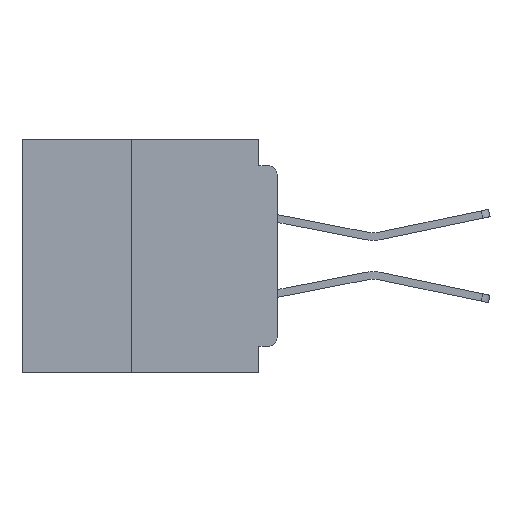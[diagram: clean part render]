
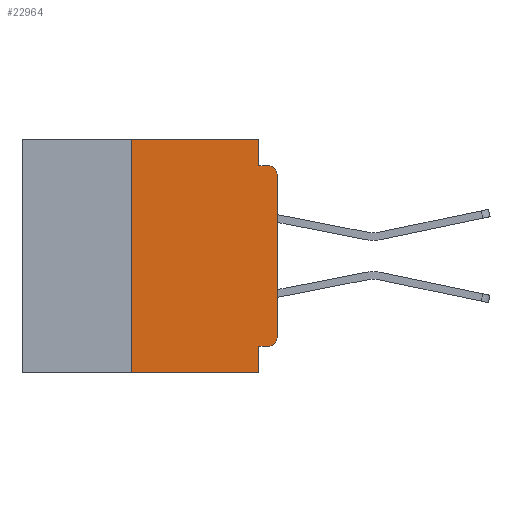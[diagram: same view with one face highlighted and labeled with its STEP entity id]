
A CAD part, left-side view. The second image highlights one B-rep face of the part: STEP entity #22964.
In plain terms, the highlighted planar face has unit normal (-1, 0, 0).
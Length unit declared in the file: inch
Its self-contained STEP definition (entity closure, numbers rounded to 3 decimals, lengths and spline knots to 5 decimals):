
#797 = ORIENTED_EDGE ( 'NONE', *, *, #20829, .T. ) ;
#1443 = DIRECTION ( 'NONE',  ( -1., 0., 0. ) ) ;
#1521 = VERTEX_POINT ( 'NONE', #8907 ) ;
#2246 = CARTESIAN_POINT ( 'NONE',  ( 0., 0.25, 0. ) ) ;
#2612 = FACE_OUTER_BOUND ( 'NONE', #40411, .T. ) ;
#3037 = DIRECTION ( 'NONE',  ( 0., 0., -1. ) ) ;
#3996 = CARTESIAN_POINT ( 'NONE',  ( 0., 0.25, -0.4 ) ) ;
#4849 = CARTESIAN_POINT ( 'NONE',  ( 0., 0.437, 0. ) ) ;
#5281 = VERTEX_POINT ( 'NONE', #40898 ) ;
#5335 = AXIS2_PLACEMENT_3D ( 'NONE', #21804, #1443, #25187 ) ;
#5814 = ORIENTED_EDGE ( 'NONE', *, *, #21959, .T. ) ;
#6691 = LINE ( 'NONE', #37808, #23656 ) ;
#6811 = LINE ( 'NONE', #42361, #14792 ) ;
#7474 = VERTEX_POINT ( 'NONE', #8950 ) ;
#7565 = CARTESIAN_POINT ( 'NONE',  ( 0., 0.031, 0. ) ) ;
#8783 = CARTESIAN_POINT ( 'NONE',  ( 0., 0.015, -0.06 ) ) ;
#8907 = CARTESIAN_POINT ( 'NONE',  ( 0., 0.25, -0.4 ) ) ;
#8950 = CARTESIAN_POINT ( 'NONE',  ( 0., 0.031, 0. ) ) ;
#9202 = VECTOR ( 'NONE', #11001, 39.37008 ) ;
#9254 = CARTESIAN_POINT ( 'NONE',  ( 0., 0.437, -0.4 ) ) ;
#9790 = LINE ( 'NONE', #35557, #41506 ) ;
#11001 = DIRECTION ( 'NONE',  ( 0., 0., -1. ) ) ;
#12199 = DIRECTION ( 'NONE',  ( 0., 0., -1. ) ) ;
#14130 = CARTESIAN_POINT ( 'NONE',  ( 0., 0.031, -0.355 ) ) ;
#14475 = VECTOR ( 'NONE', #41772, 39.37008 ) ;
#14792 = VECTOR ( 'NONE', #25555, 39.37008 ) ;
#15885 = EDGE_CURVE ( 'NONE', #7474, #5281, #28276, .T. ) ;
#16572 = PLANE ( 'NONE',  #38923 ) ;
#17125 = VERTEX_POINT ( 'NONE', #2246 ) ;
#17690 = EDGE_CURVE ( 'NONE', #39232, #34320, #42857, .T. ) ;
#18145 = CARTESIAN_POINT ( 'NONE',  ( 0., 0., 0. ) ) ;
#19674 = ORIENTED_EDGE ( 'NONE', *, *, #30195, .T. ) ;
#19969 = CARTESIAN_POINT ( 'NONE',  ( 0., 0.437, 0. ) ) ;
#20690 = VERTEX_POINT ( 'NONE', #14130 ) ;
#20829 = EDGE_CURVE ( 'NONE', #23840, #30732, #32013, .T. ) ;
#21804 = CARTESIAN_POINT ( 'NONE',  ( 0., 0.015, -0.34 ) ) ;
#21959 = EDGE_CURVE ( 'NONE', #30732, #39232, #22398, .T. ) ;
#22218 = ORIENTED_EDGE ( 'NONE', *, *, #27146, .F. ) ;
#22398 = LINE ( 'NONE', #18145, #14475 ) ;
#22964 = ADVANCED_FACE ( 'NONE', ( #2612 ), #16572, .F. ) ;
#23379 = DIRECTION ( 'NONE',  ( 1., 0., 0. ) ) ;
#23656 = VECTOR ( 'NONE', #41203, 39.37008 ) ;
#23840 = VERTEX_POINT ( 'NONE', #29068 ) ;
#24038 = VECTOR ( 'NONE', #34531, 39.37008 ) ;
#25118 = EDGE_CURVE ( 'NONE', #5281, #34320, #6811, .T. ) ;
#25187 = DIRECTION ( 'NONE',  ( 0., 0., -1. ) ) ;
#25555 = DIRECTION ( 'NONE',  ( 0., -1., 0. ) ) ;
#26166 = LINE ( 'NONE', #3996, #24038 ) ;
#26387 = LINE ( 'NONE', #4849, #27441 ) ;
#26530 = VECTOR ( 'NONE', #29518, 39.37008 ) ;
#26737 = ORIENTED_EDGE ( 'NONE', *, *, #17690, .T. ) ;
#27146 = EDGE_CURVE ( 'NONE', #23840, #20690, #6691, .T. ) ;
#27441 = VECTOR ( 'NONE', #31975, 39.37008 ) ;
#28276 = LINE ( 'NONE', #7565, #9202 ) ;
#28695 = EDGE_CURVE ( 'NONE', #1521, #17125, #26166, .T. ) ;
#28870 = ORIENTED_EDGE ( 'NONE', *, *, #25118, .F. ) ;
#29068 = CARTESIAN_POINT ( 'NONE',  ( 0., 0.015, -0.355 ) ) ;
#29518 = DIRECTION ( 'NONE',  ( 0., -1., 0. ) ) ;
#29774 = ORIENTED_EDGE ( 'NONE', *, *, #38739, .F. ) ;
#30195 = EDGE_CURVE ( 'NONE', #1521, #30522, #35515, .T. ) ;
#30522 = VERTEX_POINT ( 'NONE', #41302 ) ;
#30732 = VERTEX_POINT ( 'NONE', #39237 ) ;
#31023 = AXIS2_PLACEMENT_3D ( 'NONE', #8783, #32475, #12199 ) ;
#31975 = DIRECTION ( 'NONE',  ( 0., -1., 0. ) ) ;
#32013 = CIRCLE ( 'NONE', #5335, 0.015 ) ;
#32475 = DIRECTION ( 'NONE',  ( -1., 0., 0. ) ) ;
#33336 = ORIENTED_EDGE ( 'NONE', *, *, #40728, .F. ) ;
#34320 = VERTEX_POINT ( 'NONE', #41971 ) ;
#34531 = DIRECTION ( 'NONE',  ( 0., 0., 1. ) ) ;
#35515 = LINE ( 'NONE', #9254, #26530 ) ;
#35557 = CARTESIAN_POINT ( 'NONE',  ( 0., 0.031, -0.4 ) ) ;
#35840 = DIRECTION ( 'NONE',  ( 0., 0., -1. ) ) ;
#36409 = ORIENTED_EDGE ( 'NONE', *, *, #15885, .F. ) ;
#37808 = CARTESIAN_POINT ( 'NONE',  ( 0., 0., -0.355 ) ) ;
#37842 = CARTESIAN_POINT ( 'NONE',  ( 0., 0., -0.06 ) ) ;
#38739 = EDGE_CURVE ( 'NONE', #17125, #7474, #26387, .T. ) ;
#38923 = AXIS2_PLACEMENT_3D ( 'NONE', #19969, #23379, #3037 ) ;
#39232 = VERTEX_POINT ( 'NONE', #37842 ) ;
#39237 = CARTESIAN_POINT ( 'NONE',  ( 0., 0., -0.34 ) ) ;
#40411 = EDGE_LOOP ( 'NONE', ( #5814, #26737, #28870, #36409, #29774, #41306, #19674, #33336, #22218, #797 ) ) ;
#40728 = EDGE_CURVE ( 'NONE', #20690, #30522, #9790, .T. ) ;
#40898 = CARTESIAN_POINT ( 'NONE',  ( 0., 0.031, -0.045 ) ) ;
#41203 = DIRECTION ( 'NONE',  ( 0., 1., 0. ) ) ;
#41302 = CARTESIAN_POINT ( 'NONE',  ( 0., 0.031, -0.4 ) ) ;
#41306 = ORIENTED_EDGE ( 'NONE', *, *, #28695, .F. ) ;
#41506 = VECTOR ( 'NONE', #35840, 39.37008 ) ;
#41772 = DIRECTION ( 'NONE',  ( 0., 0., 1. ) ) ;
#41971 = CARTESIAN_POINT ( 'NONE',  ( 0., 0.015, -0.045 ) ) ;
#42361 = CARTESIAN_POINT ( 'NONE',  ( 0., 0., -0.045 ) ) ;
#42857 = CIRCLE ( 'NONE', #31023, 0.015 ) ;
